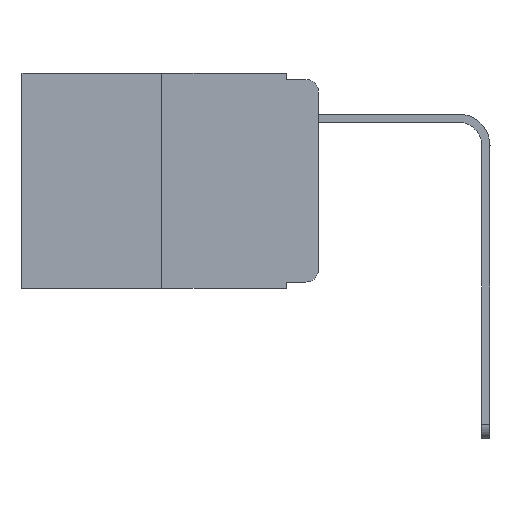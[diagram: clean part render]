
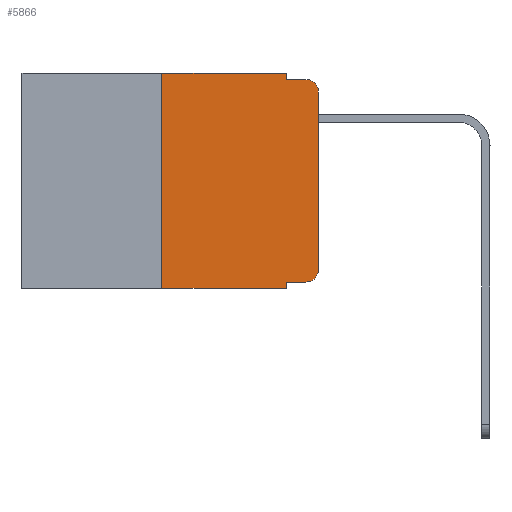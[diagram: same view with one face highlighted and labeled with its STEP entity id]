
A CAD part, left-side view. The second image highlights one B-rep face of the part: STEP entity #5866.
In plain terms, the highlighted planar face has unit normal (-1, 0, 0).
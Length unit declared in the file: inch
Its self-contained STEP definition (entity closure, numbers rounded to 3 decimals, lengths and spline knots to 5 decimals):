
#597 = EDGE_CURVE ( 'NONE', #16736, #616, #4688, .T. ) ;
#616 = VERTEX_POINT ( 'NONE', #3242 ) ;
#712 = DIRECTION ( 'NONE',  ( 0., 0., -1. ) ) ;
#1010 = DIRECTION ( 'NONE',  ( 0., 0., 1. ) ) ;
#1158 = EDGE_CURVE ( 'NONE', #12802, #16736, #13612, .T. ) ;
#1731 = VERTEX_POINT ( 'NONE', #16176 ) ;
#1739 = CARTESIAN_POINT ( 'NONE',  ( 0., 0.25, 0. ) ) ;
#1876 = ORIENTED_EDGE ( 'NONE', *, *, #18373, .T. ) ;
#2127 = VERTEX_POINT ( 'NONE', #4874 ) ;
#2546 = VECTOR ( 'NONE', #16628, 39.37008 ) ;
#2620 = VERTEX_POINT ( 'NONE', #3178 ) ;
#2845 = AXIS2_PLACEMENT_3D ( 'NONE', #8556, #15236, #8476 ) ;
#2908 = CARTESIAN_POINT ( 'NONE',  ( 0., 0.051, -0.333 ) ) ;
#3014 = VECTOR ( 'NONE', #4685, 39.37008 ) ;
#3178 = CARTESIAN_POINT ( 'NONE',  ( 0., 0., -0.03 ) ) ;
#3242 = CARTESIAN_POINT ( 'NONE',  ( 0., 0.02, -0.01 ) ) ;
#3456 = CARTESIAN_POINT ( 'NONE',  ( 0., 0.051, -0.333 ) ) ;
#4549 = VECTOR ( 'NONE', #18698, 39.37008 ) ;
#4685 = DIRECTION ( 'NONE',  ( 0., -1., 0. ) ) ;
#4688 = LINE ( 'NONE', #8220, #2546 ) ;
#4874 = CARTESIAN_POINT ( 'NONE',  ( 0., 0.051, -0.343 ) ) ;
#4886 = CIRCLE ( 'NONE', #2845, 0.02 ) ;
#4957 = LINE ( 'NONE', #15006, #5480 ) ;
#5313 = EDGE_CURVE ( 'NONE', #9101, #12802, #7732, .T. ) ;
#5327 = CARTESIAN_POINT ( 'NONE',  ( 0., 0.25, 0. ) ) ;
#5436 = DIRECTION ( 'NONE',  ( 0., -1., 0. ) ) ;
#5480 = VECTOR ( 'NONE', #20307, 39.37008 ) ;
#5565 = PLANE ( 'NONE',  #10593 ) ;
#5640 = CARTESIAN_POINT ( 'NONE',  ( 0., 0.473, 0. ) ) ;
#5813 = ORIENTED_EDGE ( 'NONE', *, *, #21638, .T. ) ;
#5815 = LINE ( 'NONE', #16305, #18197 ) ;
#5866 = ADVANCED_FACE ( 'NONE', ( #15081 ), #5565, .F. ) ;
#6441 = ORIENTED_EDGE ( 'NONE', *, *, #1158, .F. ) ;
#6939 = DIRECTION ( 'NONE',  ( -1., 0., 0. ) ) ;
#7732 = LINE ( 'NONE', #17260, #12472 ) ;
#8220 = CARTESIAN_POINT ( 'NONE',  ( 0., 0.051, -0.01 ) ) ;
#8265 = CIRCLE ( 'NONE', #12301, 0.02 ) ;
#8476 = DIRECTION ( 'NONE',  ( 0., 0., -1. ) ) ;
#8556 = CARTESIAN_POINT ( 'NONE',  ( 0., 0.02, -0.03 ) ) ;
#8565 = CARTESIAN_POINT ( 'NONE',  ( 0., 0.02, -0.313 ) ) ;
#8684 = VERTEX_POINT ( 'NONE', #9238 ) ;
#9101 = VERTEX_POINT ( 'NONE', #1739 ) ;
#9238 = CARTESIAN_POINT ( 'NONE',  ( 0., 0., -0.313 ) ) ;
#9354 = EDGE_LOOP ( 'NONE', ( #1876, #5813, #19896, #6441, #16664, #13316, #18074, #15419, #11019, #18424 ) ) ;
#9880 = CARTESIAN_POINT ( 'NONE',  ( 0., 0.051, 0. ) ) ;
#10029 = DIRECTION ( 'NONE',  ( 0., 0., -1. ) ) ;
#10593 = AXIS2_PLACEMENT_3D ( 'NONE', #5640, #20845, #10832 ) ;
#10832 = DIRECTION ( 'NONE',  ( 0., 0., -1. ) ) ;
#10862 = CARTESIAN_POINT ( 'NONE',  ( 0., 0.051, 0. ) ) ;
#11016 = CARTESIAN_POINT ( 'NONE',  ( 0., 0.051, 0. ) ) ;
#11019 = ORIENTED_EDGE ( 'NONE', *, *, #13692, .T. ) ;
#11755 = LINE ( 'NONE', #2908, #3014 ) ;
#11811 = DIRECTION ( 'NONE',  ( 0., 0., -1. ) ) ;
#11964 = LINE ( 'NONE', #5327, #4549 ) ;
#12009 = EDGE_CURVE ( 'NONE', #1731, #2127, #4957, .T. ) ;
#12301 = AXIS2_PLACEMENT_3D ( 'NONE', #8565, #6939, #11811 ) ;
#12472 = VECTOR ( 'NONE', #5436, 39.37008 ) ;
#12802 = VERTEX_POINT ( 'NONE', #11016 ) ;
#13316 = ORIENTED_EDGE ( 'NONE', *, *, #14543, .F. ) ;
#13612 = LINE ( 'NONE', #9880, #19162 ) ;
#13692 = EDGE_CURVE ( 'NONE', #18209, #16624, #11755, .T. ) ;
#14176 = CARTESIAN_POINT ( 'NONE',  ( 0., 0.02, -0.333 ) ) ;
#14285 = VECTOR ( 'NONE', #712, 39.37008 ) ;
#14543 = EDGE_CURVE ( 'NONE', #1731, #9101, #11964, .T. ) ;
#15006 = CARTESIAN_POINT ( 'NONE',  ( 0., 0.473, -0.343 ) ) ;
#15081 = FACE_OUTER_BOUND ( 'NONE', #9354, .T. ) ;
#15236 = DIRECTION ( 'NONE',  ( -1., 0., 0. ) ) ;
#15342 = EDGE_CURVE ( 'NONE', #18209, #2127, #16426, .T. ) ;
#15419 = ORIENTED_EDGE ( 'NONE', *, *, #15342, .F. ) ;
#16176 = CARTESIAN_POINT ( 'NONE',  ( 0., 0.25, -0.343 ) ) ;
#16305 = CARTESIAN_POINT ( 'NONE',  ( 0., 0., 0. ) ) ;
#16426 = LINE ( 'NONE', #10862, #14285 ) ;
#16624 = VERTEX_POINT ( 'NONE', #14176 ) ;
#16628 = DIRECTION ( 'NONE',  ( 0., -1., 0. ) ) ;
#16664 = ORIENTED_EDGE ( 'NONE', *, *, #5313, .F. ) ;
#16736 = VERTEX_POINT ( 'NONE', #19869 ) ;
#16878 = EDGE_CURVE ( 'NONE', #16624, #8684, #8265, .T. ) ;
#17260 = CARTESIAN_POINT ( 'NONE',  ( 0., 0.473, 0. ) ) ;
#18074 = ORIENTED_EDGE ( 'NONE', *, *, #12009, .T. ) ;
#18197 = VECTOR ( 'NONE', #1010, 39.37008 ) ;
#18209 = VERTEX_POINT ( 'NONE', #3456 ) ;
#18373 = EDGE_CURVE ( 'NONE', #8684, #2620, #5815, .T. ) ;
#18424 = ORIENTED_EDGE ( 'NONE', *, *, #16878, .T. ) ;
#18698 = DIRECTION ( 'NONE',  ( 0., 0., 1. ) ) ;
#19162 = VECTOR ( 'NONE', #10029, 39.37008 ) ;
#19869 = CARTESIAN_POINT ( 'NONE',  ( 0., 0.051, -0.01 ) ) ;
#19896 = ORIENTED_EDGE ( 'NONE', *, *, #597, .F. ) ;
#20307 = DIRECTION ( 'NONE',  ( 0., -1., 0. ) ) ;
#20845 = DIRECTION ( 'NONE',  ( 1., 0., 0. ) ) ;
#21638 = EDGE_CURVE ( 'NONE', #2620, #616, #4886, .T. ) ;
